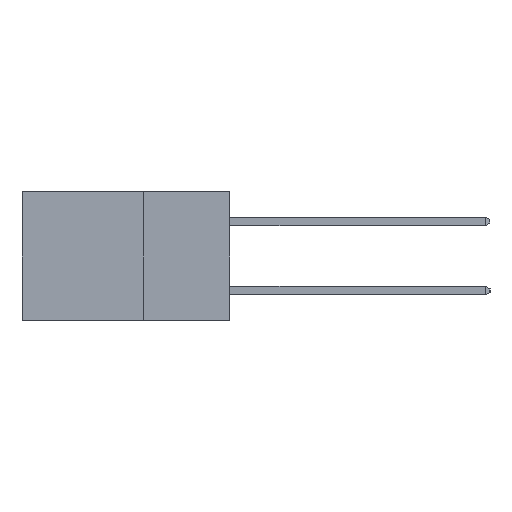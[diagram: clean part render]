
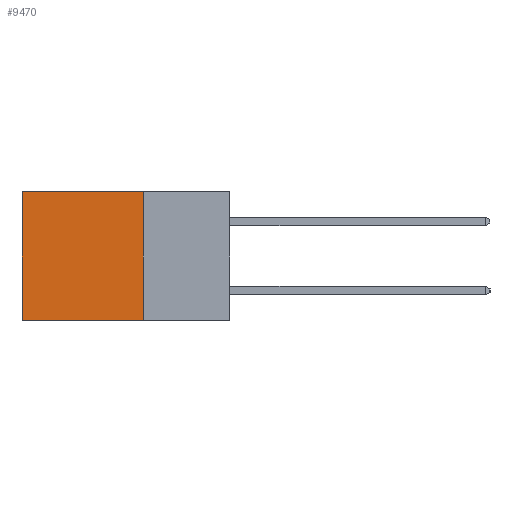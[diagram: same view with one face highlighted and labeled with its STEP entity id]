
A CAD part, left-side view. The second image highlights one B-rep face of the part: STEP entity #9470.
In plain terms, the highlighted planar face has unit normal (-1, 0, 0).
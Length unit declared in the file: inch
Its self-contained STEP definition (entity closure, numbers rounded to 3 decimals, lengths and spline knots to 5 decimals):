
#244 = VECTOR ( 'NONE', #2263, 39.37008 ) ;
#467 = CARTESIAN_POINT ( 'NONE',  ( 0.2615, 0.25, 0. ) ) ;
#645 = DIRECTION ( 'NONE',  ( 0., 1., 0. ) ) ;
#749 = VERTEX_POINT ( 'NONE', #13253 ) ;
#1018 = EDGE_CURVE ( 'NONE', #2888, #749, #8182, .T. ) ;
#1216 = FACE_OUTER_BOUND ( 'NONE', #12733, .T. ) ;
#2263 = DIRECTION ( 'NONE',  ( 0., 1., 0. ) ) ;
#2783 = PLANE ( 'NONE',  #13000 ) ;
#2888 = VERTEX_POINT ( 'NONE', #12371 ) ;
#2986 = VERTEX_POINT ( 'NONE', #7566 ) ;
#3513 = EDGE_CURVE ( 'NONE', #2986, #9957, #12888, .T. ) ;
#3621 = ORIENTED_EDGE ( 'NONE', *, *, #6541, .T. ) ;
#4139 = VECTOR ( 'NONE', #18748, 39.37008 ) ;
#4335 = DIRECTION ( 'NONE',  ( 0., 0., -1. ) ) ;
#6541 = EDGE_CURVE ( 'NONE', #2986, #2888, #8421, .T. ) ;
#7566 = CARTESIAN_POINT ( 'NONE',  ( 0.2615, 0.25, 0. ) ) ;
#7935 = VECTOR ( 'NONE', #645, 39.37008 ) ;
#8182 = LINE ( 'NONE', #8332, #12776 ) ;
#8225 = DIRECTION ( 'NONE',  ( 0., 0., -1. ) ) ;
#8332 = CARTESIAN_POINT ( 'NONE',  ( 0.2615, 0.6, -0.37 ) ) ;
#8421 = LINE ( 'NONE', #467, #7935 ) ;
#8443 = CARTESIAN_POINT ( 'NONE',  ( 0.2615, 0.25, -0.37 ) ) ;
#8550 = CARTESIAN_POINT ( 'NONE',  ( 0.2615, 0.25, -0.37 ) ) ;
#9470 = ADVANCED_FACE ( 'NONE', ( #1216 ), #2783, .F. ) ;
#9957 = VERTEX_POINT ( 'NONE', #8550 ) ;
#11150 = EDGE_CURVE ( 'NONE', #9957, #749, #16600, .T. ) ;
#12069 = CARTESIAN_POINT ( 'NONE',  ( 0.2615, 0.25, -0.37 ) ) ;
#12371 = CARTESIAN_POINT ( 'NONE',  ( 0.2615, 0.6, 0. ) ) ;
#12733 = EDGE_LOOP ( 'NONE', ( #17550, #18055, #17762, #3621 ) ) ;
#12776 = VECTOR ( 'NONE', #8225, 39.37008 ) ;
#12888 = LINE ( 'NONE', #18799, #4139 ) ;
#13000 = AXIS2_PLACEMENT_3D ( 'NONE', #12069, #13623, #4335 ) ;
#13253 = CARTESIAN_POINT ( 'NONE',  ( 0.2615, 0.6, -0.37 ) ) ;
#13623 = DIRECTION ( 'NONE',  ( 1., 0., 0. ) ) ;
#16600 = LINE ( 'NONE', #8443, #244 ) ;
#17550 = ORIENTED_EDGE ( 'NONE', *, *, #1018, .T. ) ;
#17762 = ORIENTED_EDGE ( 'NONE', *, *, #3513, .F. ) ;
#18055 = ORIENTED_EDGE ( 'NONE', *, *, #11150, .F. ) ;
#18748 = DIRECTION ( 'NONE',  ( 0., 0., -1. ) ) ;
#18799 = CARTESIAN_POINT ( 'NONE',  ( 0.2615, 0.25, -0.37 ) ) ;
